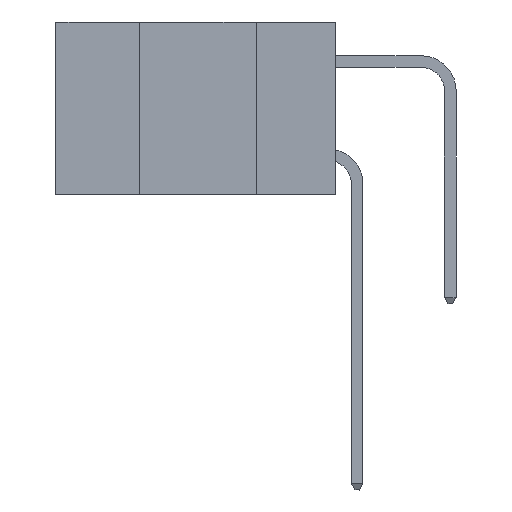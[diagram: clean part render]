
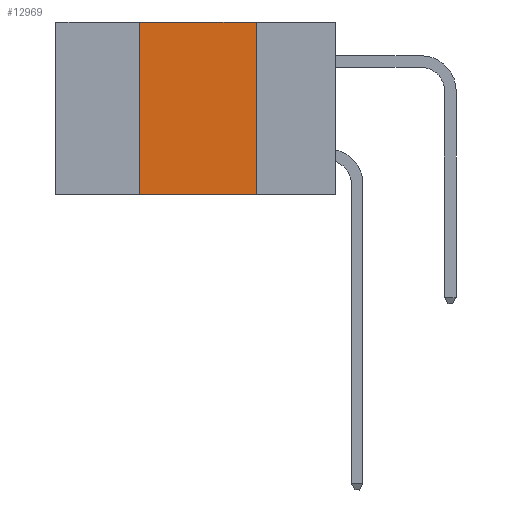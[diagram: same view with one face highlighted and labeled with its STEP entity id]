
A CAD part, left-side view. The second image highlights one B-rep face of the part: STEP entity #12969.
In plain terms, the highlighted planar face has unit normal (-1, 0, 0).
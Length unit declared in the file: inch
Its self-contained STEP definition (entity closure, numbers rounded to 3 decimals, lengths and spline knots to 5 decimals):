
#286 = ORIENTED_EDGE ( 'NONE', *, *, #17040, .F. ) ;
#636 = CARTESIAN_POINT ( 'NONE',  ( 0., 0.6, 0. ) ) ;
#798 = EDGE_LOOP ( 'NONE', ( #15556, #4937, #286, #9734 ) ) ;
#863 = VERTEX_POINT ( 'NONE', #10035 ) ;
#1454 = LINE ( 'NONE', #9678, #1560 ) ;
#1560 = VECTOR ( 'NONE', #14089, 39.37008 ) ;
#2734 = EDGE_CURVE ( 'NONE', #863, #11389, #22673, .T. ) ;
#3209 = CARTESIAN_POINT ( 'NONE',  ( 0., 0.6, -0.37 ) ) ;
#4079 = AXIS2_PLACEMENT_3D ( 'NONE', #636, #8877, #16640 ) ;
#4265 = VECTOR ( 'NONE', #11859, 39.37008 ) ;
#4287 = DIRECTION ( 'NONE',  ( 0., 0., 1. ) ) ;
#4937 = ORIENTED_EDGE ( 'NONE', *, *, #14750, .F. ) ;
#6689 = LINE ( 'NONE', #8544, #15726 ) ;
#7711 = VERTEX_POINT ( 'NONE', #20750 ) ;
#8544 = CARTESIAN_POINT ( 'NONE',  ( 0., 0.42, 0. ) ) ;
#8877 = DIRECTION ( 'NONE',  ( 1., 0., 0. ) ) ;
#9668 = CARTESIAN_POINT ( 'NONE',  ( 0., 0.17, -0.37 ) ) ;
#9678 = CARTESIAN_POINT ( 'NONE',  ( 0., 0.17, 0. ) ) ;
#9734 = ORIENTED_EDGE ( 'NONE', *, *, #2734, .T. ) ;
#10035 = CARTESIAN_POINT ( 'NONE',  ( 0., 0.42, -0.37 ) ) ;
#10943 = VECTOR ( 'NONE', #23385, 39.37008 ) ;
#11389 = VERTEX_POINT ( 'NONE', #9668 ) ;
#11859 = DIRECTION ( 'NONE',  ( 0., -1., 0. ) ) ;
#12768 = VERTEX_POINT ( 'NONE', #21817 ) ;
#12969 = ADVANCED_FACE ( 'NONE', ( #20382 ), #17682, .F. ) ;
#14089 = DIRECTION ( 'NONE',  ( 0., 0., -1. ) ) ;
#14427 = LINE ( 'NONE', #14711, #10943 ) ;
#14711 = CARTESIAN_POINT ( 'NONE',  ( 0., 0.6, 0. ) ) ;
#14750 = EDGE_CURVE ( 'NONE', #12768, #7711, #14427, .T. ) ;
#15556 = ORIENTED_EDGE ( 'NONE', *, *, #27866, .F. ) ;
#15726 = VECTOR ( 'NONE', #4287, 39.37008 ) ;
#16640 = DIRECTION ( 'NONE',  ( 0., 0., -1. ) ) ;
#17040 = EDGE_CURVE ( 'NONE', #863, #12768, #6689, .T. ) ;
#17682 = PLANE ( 'NONE',  #4079 ) ;
#20382 = FACE_OUTER_BOUND ( 'NONE', #798, .T. ) ;
#20750 = CARTESIAN_POINT ( 'NONE',  ( 0., 0.17, 0. ) ) ;
#21817 = CARTESIAN_POINT ( 'NONE',  ( 0., 0.42, 0. ) ) ;
#22673 = LINE ( 'NONE', #3209, #4265 ) ;
#23385 = DIRECTION ( 'NONE',  ( 0., -1., 0. ) ) ;
#27866 = EDGE_CURVE ( 'NONE', #7711, #11389, #1454, .T. ) ;
